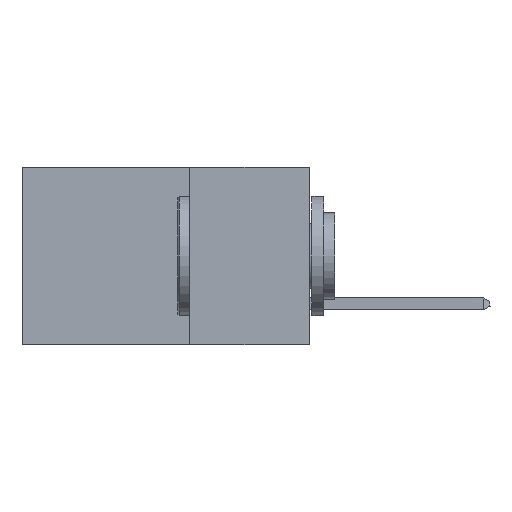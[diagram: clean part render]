
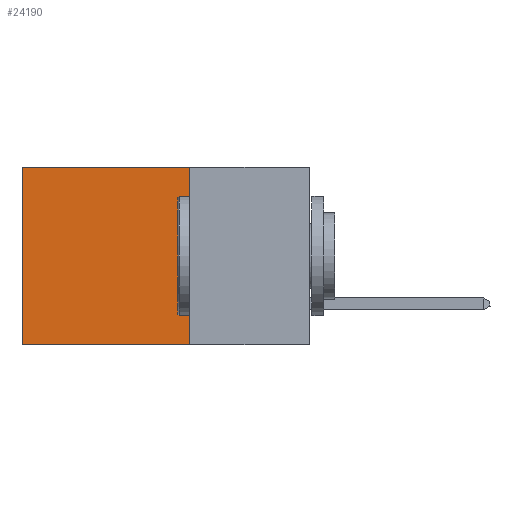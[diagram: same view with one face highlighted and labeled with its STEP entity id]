
A CAD part, left-side view. The second image highlights one B-rep face of the part: STEP entity #24190.
In plain terms, the highlighted planar face has unit normal (-1, 0, 0).
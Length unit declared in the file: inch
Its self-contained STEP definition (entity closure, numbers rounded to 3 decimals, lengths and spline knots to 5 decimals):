
#1902 = CARTESIAN_POINT ( 'NONE',  ( 0.2875, 0.6, 0. ) ) ;
#2047 = ORIENTED_EDGE ( 'NONE', *, *, #7222, .T. ) ;
#2137 = VECTOR ( 'NONE', #25596, 39.37008 ) ;
#2146 = CARTESIAN_POINT ( 'NONE',  ( 0.2875, 0.25, 0. ) ) ;
#2214 = CARTESIAN_POINT ( 'NONE',  ( 0.2875, 0.6, 0. ) ) ;
#2254 = DIRECTION ( 'NONE',  ( 0., 0., -1. ) ) ;
#2957 = VERTEX_POINT ( 'NONE', #1902 ) ;
#4117 = ORIENTED_EDGE ( 'NONE', *, *, #18269, .T. ) ;
#4250 = PLANE ( 'NONE',  #11868 ) ;
#4359 = CARTESIAN_POINT ( 'NONE',  ( 0.2875, 0.6, -0.37 ) ) ;
#4845 = DIRECTION ( 'NONE',  ( 0., 0., -1. ) ) ;
#4870 = EDGE_LOOP ( 'NONE', ( #2047, #9292, #33069, #4117 ) ) ;
#5663 = VERTEX_POINT ( 'NONE', #4359 ) ;
#6257 = CARTESIAN_POINT ( 'NONE',  ( 0.2875, 0.25, -0.37 ) ) ;
#7222 = EDGE_CURVE ( 'NONE', #2957, #5663, #31522, .T. ) ;
#9292 = ORIENTED_EDGE ( 'NONE', *, *, #9585, .F. ) ;
#9334 = DIRECTION ( 'NONE',  ( 1., 0., 0. ) ) ;
#9585 = EDGE_CURVE ( 'NONE', #12763, #5663, #26029, .T. ) ;
#9903 = CARTESIAN_POINT ( 'NONE',  ( 0.2875, 0.25, -0.37 ) ) ;
#10878 = VECTOR ( 'NONE', #4845, 39.37008 ) ;
#11205 = VECTOR ( 'NONE', #30269, 39.37008 ) ;
#11868 = AXIS2_PLACEMENT_3D ( 'NONE', #14649, #9334, #17330 ) ;
#12763 = VERTEX_POINT ( 'NONE', #6257 ) ;
#14649 = CARTESIAN_POINT ( 'NONE',  ( 0.2875, 0.25, 0. ) ) ;
#17330 = DIRECTION ( 'NONE',  ( 0., 0., -1. ) ) ;
#17686 = LINE ( 'NONE', #2146, #21291 ) ;
#18269 = EDGE_CURVE ( 'NONE', #19359, #2957, #23219, .T. ) ;
#19098 = CARTESIAN_POINT ( 'NONE',  ( 0.2875, 0.25, 0. ) ) ;
#19359 = VERTEX_POINT ( 'NONE', #19098 ) ;
#21291 = VECTOR ( 'NONE', #2254, 39.37008 ) ;
#23219 = LINE ( 'NONE', #27617, #11205 ) ;
#24190 = ADVANCED_FACE ( 'NONE', ( #28289 ), #4250, .F. ) ;
#25596 = DIRECTION ( 'NONE',  ( 0., 1., 0. ) ) ;
#26029 = LINE ( 'NONE', #9903, #2137 ) ;
#27617 = CARTESIAN_POINT ( 'NONE',  ( 0.2875, 0.25, 0. ) ) ;
#28289 = FACE_OUTER_BOUND ( 'NONE', #4870, .T. ) ;
#30269 = DIRECTION ( 'NONE',  ( 0., 1., 0. ) ) ;
#31522 = LINE ( 'NONE', #2214, #10878 ) ;
#32603 = EDGE_CURVE ( 'NONE', #19359, #12763, #17686, .T. ) ;
#33069 = ORIENTED_EDGE ( 'NONE', *, *, #32603, .F. ) ;
